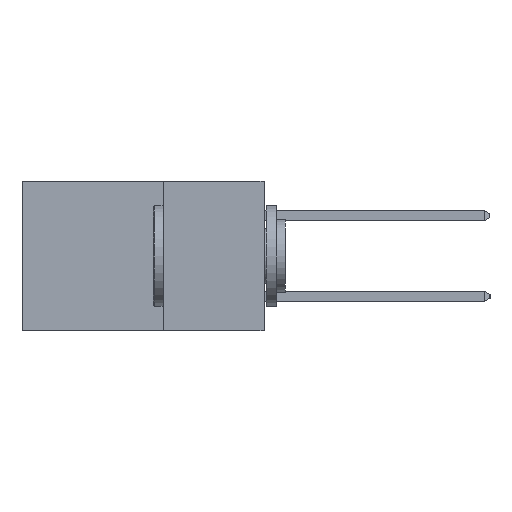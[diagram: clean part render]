
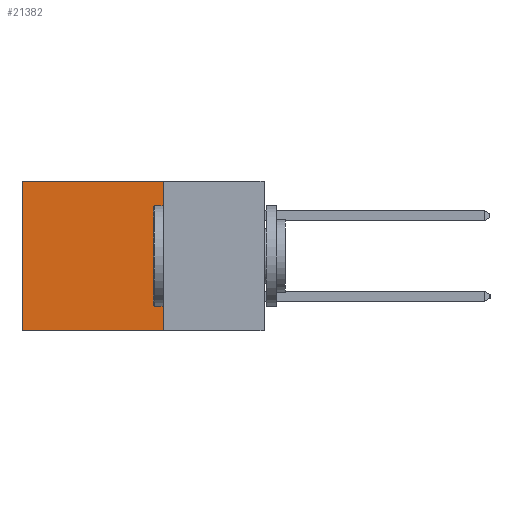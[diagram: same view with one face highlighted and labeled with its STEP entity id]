
A CAD part, left-side view. The second image highlights one B-rep face of the part: STEP entity #21382.
In plain terms, the highlighted planar face has unit normal (-1, 0, 0).
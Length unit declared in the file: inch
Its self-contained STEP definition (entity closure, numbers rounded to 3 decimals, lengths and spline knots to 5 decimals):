
#316 = ORIENTED_EDGE ( 'NONE', *, *, #10019, .F. ) ;
#468 = VECTOR ( 'NONE', #17009, 39.37008 ) ;
#607 = ORIENTED_EDGE ( 'NONE', *, *, #15668, .F. ) ;
#688 = VERTEX_POINT ( 'NONE', #14824 ) ;
#1061 = VECTOR ( 'NONE', #10986, 39.37008 ) ;
#2718 = CARTESIAN_POINT ( 'NONE',  ( 0.2615, 0.6, -0.37 ) ) ;
#4154 = PLANE ( 'NONE',  #21820 ) ;
#4620 = CARTESIAN_POINT ( 'NONE',  ( 0.2615, 0.6, 0. ) ) ;
#4832 = CARTESIAN_POINT ( 'NONE',  ( 0.2615, 0.25, -0.37 ) ) ;
#6074 = VERTEX_POINT ( 'NONE', #20635 ) ;
#6170 = DIRECTION ( 'NONE',  ( 0., 0., -1. ) ) ;
#6182 = CARTESIAN_POINT ( 'NONE',  ( 0.2615, 0.25, 0. ) ) ;
#6441 = EDGE_CURVE ( 'NONE', #688, #18043, #20201, .T. ) ;
#6696 = VERTEX_POINT ( 'NONE', #4832 ) ;
#7654 = VECTOR ( 'NONE', #22189, 39.37008 ) ;
#8930 = LINE ( 'NONE', #2718, #7654 ) ;
#9920 = EDGE_CURVE ( 'NONE', #18043, #6074, #8930, .T. ) ;
#10019 = EDGE_CURVE ( 'NONE', #6696, #6074, #23011, .T. ) ;
#10089 = CARTESIAN_POINT ( 'NONE',  ( 0.2615, 0.25, -0.37 ) ) ;
#10642 = VECTOR ( 'NONE', #19694, 39.37008 ) ;
#10986 = DIRECTION ( 'NONE',  ( 0., 1., 0. ) ) ;
#14482 = ORIENTED_EDGE ( 'NONE', *, *, #9920, .T. ) ;
#14736 = CARTESIAN_POINT ( 'NONE',  ( 0.2615, 0.25, -0.37 ) ) ;
#14824 = CARTESIAN_POINT ( 'NONE',  ( 0.2615, 0.25, 0. ) ) ;
#15668 = EDGE_CURVE ( 'NONE', #688, #6696, #21255, .T. ) ;
#17009 = DIRECTION ( 'NONE',  ( 0., 0., -1. ) ) ;
#17776 = DIRECTION ( 'NONE',  ( 1., 0., 0. ) ) ;
#18043 = VERTEX_POINT ( 'NONE', #4620 ) ;
#18715 = ORIENTED_EDGE ( 'NONE', *, *, #6441, .T. ) ;
#19145 = EDGE_LOOP ( 'NONE', ( #14482, #316, #607, #18715 ) ) ;
#19694 = DIRECTION ( 'NONE',  ( 0., 1., 0. ) ) ;
#20201 = LINE ( 'NONE', #6182, #10642 ) ;
#20635 = CARTESIAN_POINT ( 'NONE',  ( 0.2615, 0.6, -0.37 ) ) ;
#20867 = CARTESIAN_POINT ( 'NONE',  ( 0.2615, 0.25, -0.37 ) ) ;
#21255 = LINE ( 'NONE', #20867, #468 ) ;
#21382 = ADVANCED_FACE ( 'NONE', ( #24016 ), #4154, .F. ) ;
#21820 = AXIS2_PLACEMENT_3D ( 'NONE', #10089, #17776, #6170 ) ;
#22189 = DIRECTION ( 'NONE',  ( 0., 0., -1. ) ) ;
#23011 = LINE ( 'NONE', #14736, #1061 ) ;
#24016 = FACE_OUTER_BOUND ( 'NONE', #19145, .T. ) ;
